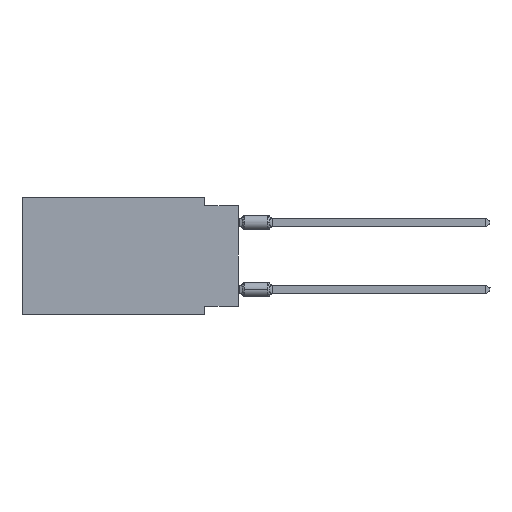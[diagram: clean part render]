
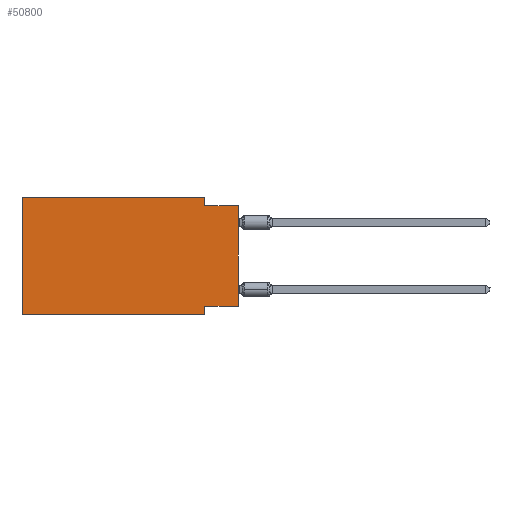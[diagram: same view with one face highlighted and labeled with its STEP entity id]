
A CAD part, left-side view. The second image highlights one B-rep face of the part: STEP entity #50800.
In plain terms, the highlighted planar face has unit normal (-1, 0, 0).
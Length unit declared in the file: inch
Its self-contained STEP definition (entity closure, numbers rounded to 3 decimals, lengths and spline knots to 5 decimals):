
#687 = DIRECTION ( 'NONE',  ( 0., -1., 0. ) ) ;
#1798 = CARTESIAN_POINT ( 'NONE',  ( 0., 0.645, 0. ) ) ;
#2347 = VECTOR ( 'NONE', #38322, 39.37008 ) ;
#2956 = VERTEX_POINT ( 'NONE', #32676 ) ;
#4752 = CARTESIAN_POINT ( 'NONE',  ( 0., 0., -0.325 ) ) ;
#9493 = CARTESIAN_POINT ( 'NONE',  ( 0., 0.645, 0. ) ) ;
#11209 = VERTEX_POINT ( 'NONE', #42657 ) ;
#11302 = DIRECTION ( 'NONE',  ( 1., 0., 0. ) ) ;
#13802 = EDGE_CURVE ( 'NONE', #11209, #2956, #22995, .T. ) ;
#14297 = EDGE_CURVE ( 'NONE', #51519, #2956, #50470, .T. ) ;
#15790 = VECTOR ( 'NONE', #687, 39.37008 ) ;
#16755 = EDGE_CURVE ( 'NONE', #32228, #48227, #50746, .T. ) ;
#17027 = LINE ( 'NONE', #32735, #2347 ) ;
#17305 = ORIENTED_EDGE ( 'NONE', *, *, #20207, .F. ) ;
#17435 = DIRECTION ( 'NONE',  ( 0., -1., 0. ) ) ;
#17810 = DIRECTION ( 'NONE',  ( 0., 0., -1. ) ) ;
#17860 = LINE ( 'NONE', #1798, #45843 ) ;
#19055 = VERTEX_POINT ( 'NONE', #20371 ) ;
#20207 = EDGE_CURVE ( 'NONE', #48227, #11209, #60667, .T. ) ;
#20371 = CARTESIAN_POINT ( 'NONE',  ( 0., 0.645, -0.35 ) ) ;
#22995 = LINE ( 'NONE', #65163, #23943 ) ;
#23534 = DIRECTION ( 'NONE',  ( 0., -1., 0. ) ) ;
#23943 = VECTOR ( 'NONE', #17435, 39.37008 ) ;
#24285 = CARTESIAN_POINT ( 'NONE',  ( 0., 0., 0. ) ) ;
#25194 = ORIENTED_EDGE ( 'NONE', *, *, #41648, .F. ) ;
#26286 = ORIENTED_EDGE ( 'NONE', *, *, #37275, .F. ) ;
#27213 = ORIENTED_EDGE ( 'NONE', *, *, #16755, .F. ) ;
#27932 = CARTESIAN_POINT ( 'NONE',  ( 0., 0.1, 0. ) ) ;
#28076 = CARTESIAN_POINT ( 'NONE',  ( 0., 0.1, -0.325 ) ) ;
#31141 = CARTESIAN_POINT ( 'NONE',  ( 0., 0.1, -0.35 ) ) ;
#32228 = VERTEX_POINT ( 'NONE', #44146 ) ;
#32582 = DIRECTION ( 'NONE',  ( 0., 0., -1. ) ) ;
#32676 = CARTESIAN_POINT ( 'NONE',  ( 0., 0., -0.025 ) ) ;
#32735 = CARTESIAN_POINT ( 'NONE',  ( 0., 0.1, -0.35 ) ) ;
#36524 = CARTESIAN_POINT ( 'NONE',  ( 0., 0.1, 0. ) ) ;
#37275 = EDGE_CURVE ( 'NONE', #42485, #65036, #17027, .T. ) ;
#37642 = EDGE_CURVE ( 'NONE', #19055, #65036, #53060, .T. ) ;
#38322 = DIRECTION ( 'NONE',  ( 0., 0., -1. ) ) ;
#39817 = DIRECTION ( 'NONE',  ( 0., 0., 1. ) ) ;
#39878 = ORIENTED_EDGE ( 'NONE', *, *, #55552, .F. ) ;
#39937 = AXIS2_PLACEMENT_3D ( 'NONE', #64289, #11302, #32582 ) ;
#40008 = DIRECTION ( 'NONE',  ( 0., 0., 1. ) ) ;
#41026 = ORIENTED_EDGE ( 'NONE', *, *, #37642, .T. ) ;
#41648 = EDGE_CURVE ( 'NONE', #19055, #32228, #17860, .T. ) ;
#42485 = VERTEX_POINT ( 'NONE', #28076 ) ;
#42657 = CARTESIAN_POINT ( 'NONE',  ( 0., 0.1, -0.025 ) ) ;
#43029 = VECTOR ( 'NONE', #23534, 39.37008 ) ;
#44146 = CARTESIAN_POINT ( 'NONE',  ( 0., 0.645, 0. ) ) ;
#45126 = CARTESIAN_POINT ( 'NONE',  ( 0., 0., -0.325 ) ) ;
#45843 = VECTOR ( 'NONE', #39817, 39.37008 ) ;
#47816 = VECTOR ( 'NONE', #17810, 39.37008 ) ;
#48227 = VERTEX_POINT ( 'NONE', #36524 ) ;
#50470 = LINE ( 'NONE', #24285, #58558 ) ;
#50746 = LINE ( 'NONE', #9493, #43029 ) ;
#50800 = ADVANCED_FACE ( 'NONE', ( #58068 ), #63959, .F. ) ;
#51519 = VERTEX_POINT ( 'NONE', #45126 ) ;
#51832 = DIRECTION ( 'NONE',  ( 0., 1., 0. ) ) ;
#53060 = LINE ( 'NONE', #54061, #15790 ) ;
#53087 = VECTOR ( 'NONE', #51832, 39.37008 ) ;
#54061 = CARTESIAN_POINT ( 'NONE',  ( 0., 0.645, -0.35 ) ) ;
#54428 = ORIENTED_EDGE ( 'NONE', *, *, #14297, .T. ) ;
#55552 = EDGE_CURVE ( 'NONE', #51519, #42485, #68176, .T. ) ;
#58068 = FACE_OUTER_BOUND ( 'NONE', #63634, .T. ) ;
#58558 = VECTOR ( 'NONE', #40008, 39.37008 ) ;
#60667 = LINE ( 'NONE', #27932, #47816 ) ;
#63634 = EDGE_LOOP ( 'NONE', ( #54428, #65694, #17305, #27213, #25194, #41026, #26286, #39878 ) ) ;
#63959 = PLANE ( 'NONE',  #39937 ) ;
#64289 = CARTESIAN_POINT ( 'NONE',  ( 0., 0.645, 0. ) ) ;
#65036 = VERTEX_POINT ( 'NONE', #31141 ) ;
#65163 = CARTESIAN_POINT ( 'NONE',  ( 0., 0., -0.025 ) ) ;
#65694 = ORIENTED_EDGE ( 'NONE', *, *, #13802, .F. ) ;
#68176 = LINE ( 'NONE', #4752, #53087 ) ;
